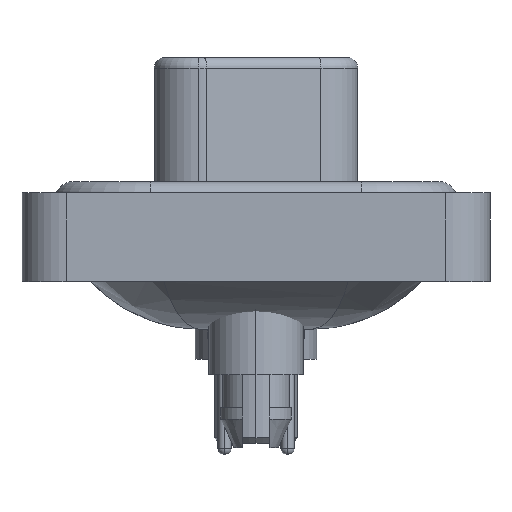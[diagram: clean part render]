
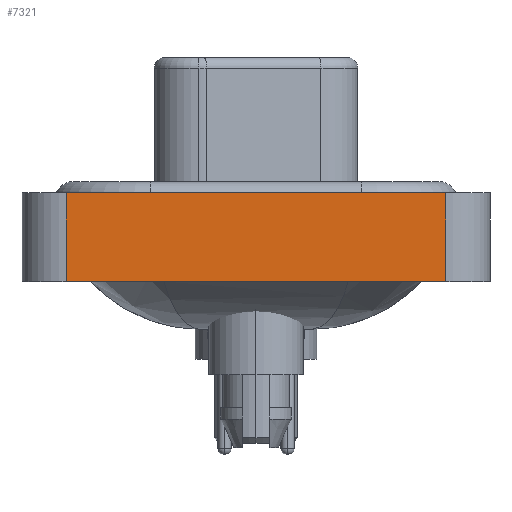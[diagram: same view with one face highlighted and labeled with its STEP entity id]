
A CAD part, left-side view. The second image highlights one B-rep face of the part: STEP entity #7321.
In plain terms, the highlighted planar face has unit normal (-1, 0, 0).
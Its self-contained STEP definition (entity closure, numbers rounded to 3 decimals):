
#77 = AXIS2_PLACEMENT_3D ( 'NONE', #19358, #266, #7137 ) ;
#266 = DIRECTION ( 'NONE',  ( -1., 0., 0. ) ) ;
#1853 = CARTESIAN_POINT ( 'NONE',  ( -7.25, -8.55, -3.6 ) ) ;
#2023 = VERTEX_POINT ( 'NONE', #15493 ) ;
#2369 = EDGE_CURVE ( 'NONE', #2023, #19704, #15583, .T. ) ;
#3024 = CARTESIAN_POINT ( 'NONE',  ( -7.25, -8.55, -3.6 ) ) ;
#3944 = VERTEX_POINT ( 'NONE', #19509 ) ;
#4618 = EDGE_CURVE ( 'NONE', #19704, #11611, #15334, .T. ) ;
#7137 = DIRECTION ( 'NONE',  ( 0., 0., 1. ) ) ;
#7321 = ADVANCED_FACE ( 'NONE', ( #19585 ), #15917, .T. ) ;
#8729 = DIRECTION ( 'NONE',  ( 0., 0., 1. ) ) ;
#10612 = CARTESIAN_POINT ( 'NONE',  ( -7.25, -8.55, 0.4 ) ) ;
#11060 = ORIENTED_EDGE ( 'NONE', *, *, #4618, .T. ) ;
#11611 = VERTEX_POINT ( 'NONE', #13587 ) ;
#11634 = VECTOR ( 'NONE', #8729, 1000. ) ;
#12636 = ORIENTED_EDGE ( 'NONE', *, *, #2369, .T. ) ;
#12857 = VECTOR ( 'NONE', #22580, 1000. ) ;
#13174 = EDGE_LOOP ( 'NONE', ( #11060, #14144, #14832, #12636 ) ) ;
#13587 = CARTESIAN_POINT ( 'NONE',  ( -7.25, -8.55, 0.4 ) ) ;
#14144 = ORIENTED_EDGE ( 'NONE', *, *, #18659, .F. ) ;
#14832 = ORIENTED_EDGE ( 'NONE', *, *, #17600, .F. ) ;
#15225 = DIRECTION ( 'NONE',  ( 0., 0., 1. ) ) ;
#15334 = LINE ( 'NONE', #20498, #17713 ) ;
#15493 = CARTESIAN_POINT ( 'NONE',  ( -7.25, 8.55, -3.6 ) ) ;
#15583 = LINE ( 'NONE', #1853, #12857 ) ;
#15917 = PLANE ( 'NONE',  #77 ) ;
#15966 = DIRECTION ( 'NONE',  ( 0., -1., 0. ) ) ;
#17526 = LINE ( 'NONE', #18801, #11634 ) ;
#17600 = EDGE_CURVE ( 'NONE', #2023, #3944, #17526, .T. ) ;
#17713 = VECTOR ( 'NONE', #15225, 1000. ) ;
#18659 = EDGE_CURVE ( 'NONE', #3944, #11611, #21132, .T. ) ;
#18801 = CARTESIAN_POINT ( 'NONE',  ( -7.25, 8.55, -3.6 ) ) ;
#19358 = CARTESIAN_POINT ( 'NONE',  ( -7.25, -8.55, -3.6 ) ) ;
#19509 = CARTESIAN_POINT ( 'NONE',  ( -7.25, 8.55, 0.4 ) ) ;
#19585 = FACE_OUTER_BOUND ( 'NONE', #13174, .T. ) ;
#19704 = VERTEX_POINT ( 'NONE', #3024 ) ;
#20498 = CARTESIAN_POINT ( 'NONE',  ( -7.25, -8.55, -3.6 ) ) ;
#21132 = LINE ( 'NONE', #10612, #21186 ) ;
#21186 = VECTOR ( 'NONE', #15966, 1000. ) ;
#22580 = DIRECTION ( 'NONE',  ( 0., -1., 0. ) ) ;
